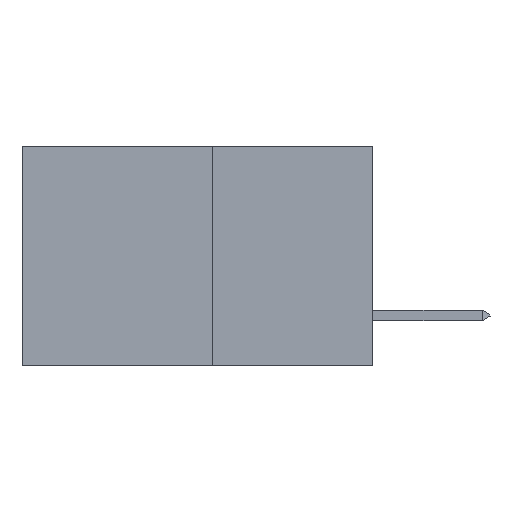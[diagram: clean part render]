
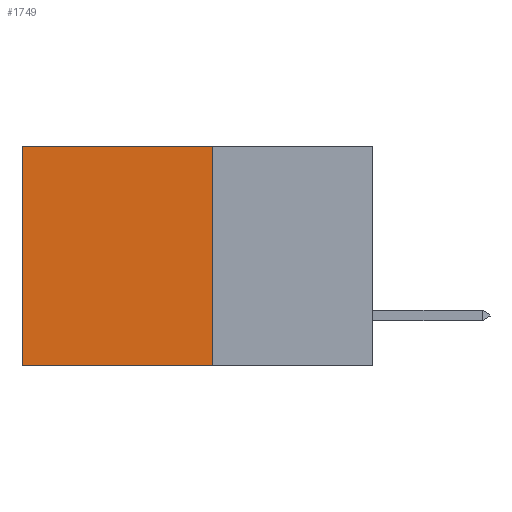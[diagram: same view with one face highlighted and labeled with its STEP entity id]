
A CAD part, left-side view. The second image highlights one B-rep face of the part: STEP entity #1749.
In plain terms, the highlighted planar face has unit normal (-1, 0, 0).
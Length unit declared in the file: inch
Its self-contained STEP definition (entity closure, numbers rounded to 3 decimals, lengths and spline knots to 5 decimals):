
#1137 = CARTESIAN_POINT ( 'NONE',  ( 0.277, 0.59, 0. ) ) ;
#1356 = AXIS2_PLACEMENT_3D ( 'NONE', #4341, #12619, #12638 ) ;
#1429 = PLANE ( 'NONE',  #1356 ) ;
#1676 = LINE ( 'NONE', #15586, #15179 ) ;
#1749 = ADVANCED_FACE ( 'NONE', ( #12166 ), #1429, .F. ) ;
#1758 = ORIENTED_EDGE ( 'NONE', *, *, #11394, .T. ) ;
#2591 = EDGE_CURVE ( 'NONE', #8688, #14731, #1676, .T. ) ;
#2956 = CARTESIAN_POINT ( 'NONE',  ( 0.277, 0.27, -0.37 ) ) ;
#3688 = ORIENTED_EDGE ( 'NONE', *, *, #12816, .F. ) ;
#4341 = CARTESIAN_POINT ( 'NONE',  ( 0.277, 0.27, -0.37 ) ) ;
#5365 = ORIENTED_EDGE ( 'NONE', *, *, #7345, .F. ) ;
#5471 = CARTESIAN_POINT ( 'NONE',  ( 0.277, 0.59, -0.37 ) ) ;
#5928 = DIRECTION ( 'NONE',  ( 0., 1., 0. ) ) ;
#6192 = CARTESIAN_POINT ( 'NONE',  ( 0.277, 0.27, -0.37 ) ) ;
#7272 = VERTEX_POINT ( 'NONE', #2956 ) ;
#7345 = EDGE_CURVE ( 'NONE', #8688, #7272, #7827, .T. ) ;
#7440 = DIRECTION ( 'NONE',  ( 0., 0., -1. ) ) ;
#7827 = LINE ( 'NONE', #6192, #11357 ) ;
#8688 = VERTEX_POINT ( 'NONE', #11542 ) ;
#9272 = DIRECTION ( 'NONE',  ( 0., 0., -1. ) ) ;
#9411 = VERTEX_POINT ( 'NONE', #15595 ) ;
#10570 = VECTOR ( 'NONE', #9272, 39.37008 ) ;
#10875 = DIRECTION ( 'NONE',  ( 0., 1., 0. ) ) ;
#11357 = VECTOR ( 'NONE', #7440, 39.37008 ) ;
#11394 = EDGE_CURVE ( 'NONE', #14731, #9411, #14101, .T. ) ;
#11542 = CARTESIAN_POINT ( 'NONE',  ( 0.277, 0.27, 0. ) ) ;
#11991 = LINE ( 'NONE', #16331, #15046 ) ;
#12123 = EDGE_LOOP ( 'NONE', ( #1758, #3688, #5365, #14557 ) ) ;
#12166 = FACE_OUTER_BOUND ( 'NONE', #12123, .T. ) ;
#12619 = DIRECTION ( 'NONE',  ( 1., 0., 0. ) ) ;
#12638 = DIRECTION ( 'NONE',  ( 0., 0., -1. ) ) ;
#12816 = EDGE_CURVE ( 'NONE', #7272, #9411, #11991, .T. ) ;
#14101 = LINE ( 'NONE', #5471, #10570 ) ;
#14557 = ORIENTED_EDGE ( 'NONE', *, *, #2591, .T. ) ;
#14731 = VERTEX_POINT ( 'NONE', #1137 ) ;
#15046 = VECTOR ( 'NONE', #5928, 39.37008 ) ;
#15179 = VECTOR ( 'NONE', #10875, 39.37008 ) ;
#15586 = CARTESIAN_POINT ( 'NONE',  ( 0.277, 0.27, 0. ) ) ;
#15595 = CARTESIAN_POINT ( 'NONE',  ( 0.277, 0.59, -0.37 ) ) ;
#16331 = CARTESIAN_POINT ( 'NONE',  ( 0.277, 0.27, -0.37 ) ) ;
